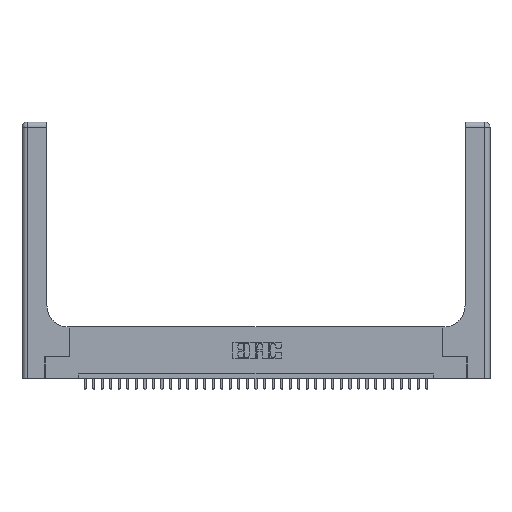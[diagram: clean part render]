
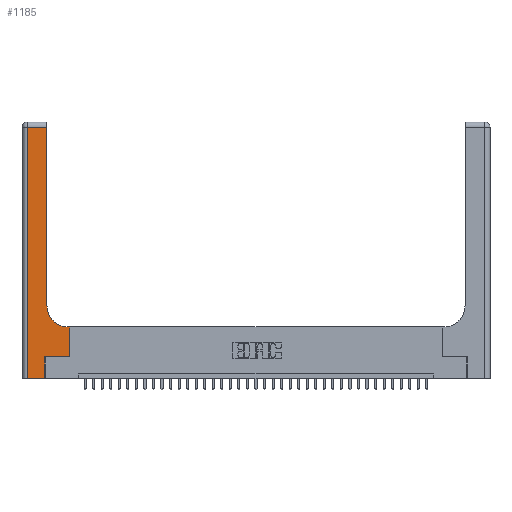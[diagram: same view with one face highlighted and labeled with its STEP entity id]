
A CAD part, top view. The second image highlights one B-rep face of the part: STEP entity #1185.
In plain terms, the highlighted planar face has unit normal (0, 0, 1).
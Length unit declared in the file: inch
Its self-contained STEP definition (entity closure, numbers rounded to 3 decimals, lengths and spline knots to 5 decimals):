
#164 = VECTOR ( 'NONE', #12510, 39.37008 ) ;
#428 = CARTESIAN_POINT ( 'NONE',  ( 0.06, 2.94, 0.37 ) ) ;
#627 = ORIENTED_EDGE ( 'NONE', *, *, #19803, .T. ) ;
#870 = CARTESIAN_POINT ( 'NONE',  ( 0.5415, 0.6, 0.37 ) ) ;
#956 = EDGE_CURVE ( 'NONE', #2668, #35940, #22018, .T. ) ;
#964 = DIRECTION ( 'NONE',  ( -1., 0., 0. ) ) ;
#1028 = LINE ( 'NONE', #12413, #24579 ) ;
#1185 = ADVANCED_FACE ( 'NONE', ( #35589 ), #9181, .F. ) ;
#1253 = CARTESIAN_POINT ( 'NONE',  ( 0., 0., 0.37 ) ) ;
#1738 = VERTEX_POINT ( 'NONE', #20314 ) ;
#1837 = VECTOR ( 'NONE', #16907, 39.37008 ) ;
#2039 = EDGE_CURVE ( 'NONE', #35940, #33657, #1028, .T. ) ;
#2090 = EDGE_CURVE ( 'NONE', #4696, #23273, #7519, .T. ) ;
#2668 = VERTEX_POINT ( 'NONE', #35515 ) ;
#3019 = ORIENTED_EDGE ( 'NONE', *, *, #16258, .T. ) ;
#3711 = DIRECTION ( 'NONE',  ( 0., 0., -1. ) ) ;
#3886 = ORIENTED_EDGE ( 'NONE', *, *, #2039, .T. ) ;
#4696 = VERTEX_POINT ( 'NONE', #870 ) ;
#6920 = AXIS2_PLACEMENT_3D ( 'NONE', #28801, #11972, #964 ) ;
#6997 = VECTOR ( 'NONE', #17640, 39.37008 ) ;
#7273 = EDGE_CURVE ( 'NONE', #19159, #4696, #32835, .T. ) ;
#7519 = CIRCLE ( 'NONE', #21207, 0.25 ) ;
#7888 = VECTOR ( 'NONE', #30811, 39.37008 ) ;
#7930 = CARTESIAN_POINT ( 'NONE',  ( 0.2915, 0.85, 0.37 ) ) ;
#8381 = CARTESIAN_POINT ( 'NONE',  ( 0.5585, 0.25, 0.37 ) ) ;
#9181 = PLANE ( 'NONE',  #6920 ) ;
#9701 = EDGE_LOOP ( 'NONE', ( #3019, #19278, #11784, #17271, #23940, #3886, #627, #13841, #27647 ) ) ;
#11057 = EDGE_CURVE ( 'NONE', #1738, #2668, #17279, .T. ) ;
#11254 = CARTESIAN_POINT ( 'NONE',  ( 0.06, 3., 0.37 ) ) ;
#11784 = ORIENTED_EDGE ( 'NONE', *, *, #15446, .T. ) ;
#11972 = DIRECTION ( 'NONE',  ( 0., 0., -1. ) ) ;
#12272 = CARTESIAN_POINT ( 'NONE',  ( 0.5585, 0.6, 0.37 ) ) ;
#12413 = CARTESIAN_POINT ( 'NONE',  ( 0.269, 0.25, 0.37 ) ) ;
#12494 = VECTOR ( 'NONE', #28352, 39.37008 ) ;
#12510 = DIRECTION ( 'NONE',  ( 0., 1., 0. ) ) ;
#13841 = ORIENTED_EDGE ( 'NONE', *, *, #7273, .T. ) ;
#13890 = LINE ( 'NONE', #28261, #20987 ) ;
#15446 = EDGE_CURVE ( 'NONE', #25880, #1738, #21019, .T. ) ;
#16258 = EDGE_CURVE ( 'NONE', #23273, #16773, #34852, .T. ) ;
#16773 = VERTEX_POINT ( 'NONE', #25052 ) ;
#16907 = DIRECTION ( 'NONE',  ( 0., 1., 0. ) ) ;
#17080 = DIRECTION ( 'NONE',  ( -1., 0., 0. ) ) ;
#17271 = ORIENTED_EDGE ( 'NONE', *, *, #11057, .T. ) ;
#17279 = LINE ( 'NONE', #1253, #31865 ) ;
#17548 = CARTESIAN_POINT ( 'NONE',  ( 0.5415, 0.85, 0.37 ) ) ;
#17640 = DIRECTION ( 'NONE',  ( -1., 0., 0. ) ) ;
#17679 = DIRECTION ( 'NONE',  ( 1., 0., 0. ) ) ;
#19159 = VERTEX_POINT ( 'NONE', #12272 ) ;
#19278 = ORIENTED_EDGE ( 'NONE', *, *, #24133, .T. ) ;
#19803 = EDGE_CURVE ( 'NONE', #33657, #19159, #21893, .T. ) ;
#20314 = CARTESIAN_POINT ( 'NONE',  ( 0.06, 0., 0.37 ) ) ;
#20861 = DIRECTION ( 'NONE',  ( 1., 0., 0. ) ) ;
#20987 = VECTOR ( 'NONE', #17080, 39.37008 ) ;
#21019 = LINE ( 'NONE', #11254, #7888 ) ;
#21207 = AXIS2_PLACEMENT_3D ( 'NONE', #17548, #3711, #26027 ) ;
#21893 = LINE ( 'NONE', #31282, #1837 ) ;
#22018 = LINE ( 'NONE', #26133, #164 ) ;
#23273 = VERTEX_POINT ( 'NONE', #7930 ) ;
#23940 = ORIENTED_EDGE ( 'NONE', *, *, #956, .T. ) ;
#24133 = EDGE_CURVE ( 'NONE', #16773, #25880, #13890, .T. ) ;
#24579 = VECTOR ( 'NONE', #17679, 39.37008 ) ;
#25052 = CARTESIAN_POINT ( 'NONE',  ( 0.2915, 2.94, 0.37 ) ) ;
#25880 = VERTEX_POINT ( 'NONE', #428 ) ;
#26027 = DIRECTION ( 'NONE',  ( 1., 0., 0. ) ) ;
#26133 = CARTESIAN_POINT ( 'NONE',  ( 0.269, 0., 0.37 ) ) ;
#27647 = ORIENTED_EDGE ( 'NONE', *, *, #2090, .T. ) ;
#27890 = CARTESIAN_POINT ( 'NONE',  ( 0.2915, 3., 0.37 ) ) ;
#28261 = CARTESIAN_POINT ( 'NONE',  ( 0., 2.94, 0.37 ) ) ;
#28352 = DIRECTION ( 'NONE',  ( 0., 1., 0. ) ) ;
#28801 = CARTESIAN_POINT ( 'NONE',  ( 0., 3., 0.37 ) ) ;
#30811 = DIRECTION ( 'NONE',  ( 0., -1., 0. ) ) ;
#31155 = CARTESIAN_POINT ( 'NONE',  ( 0.269, 0.25, 0.37 ) ) ;
#31282 = CARTESIAN_POINT ( 'NONE',  ( 0.5585, 0.25, 0.37 ) ) ;
#31518 = CARTESIAN_POINT ( 'NONE',  ( 0.2915, 0.6, 0.37 ) ) ;
#31865 = VECTOR ( 'NONE', #20861, 39.37008 ) ;
#32835 = LINE ( 'NONE', #31518, #6997 ) ;
#33657 = VERTEX_POINT ( 'NONE', #8381 ) ;
#34852 = LINE ( 'NONE', #27890, #12494 ) ;
#35515 = CARTESIAN_POINT ( 'NONE',  ( 0.269, 0., 0.37 ) ) ;
#35589 = FACE_OUTER_BOUND ( 'NONE', #9701, .T. ) ;
#35940 = VERTEX_POINT ( 'NONE', #31155 ) ;
